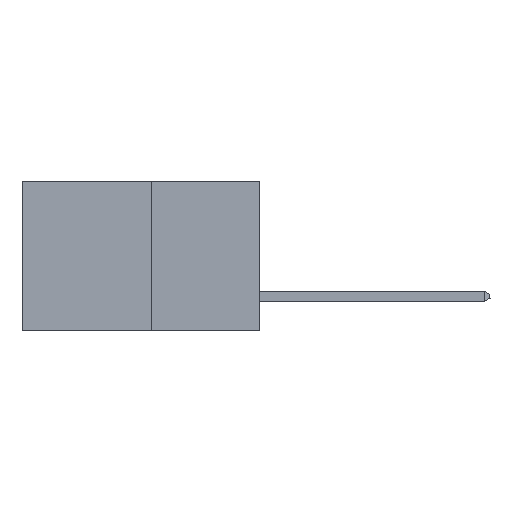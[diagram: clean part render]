
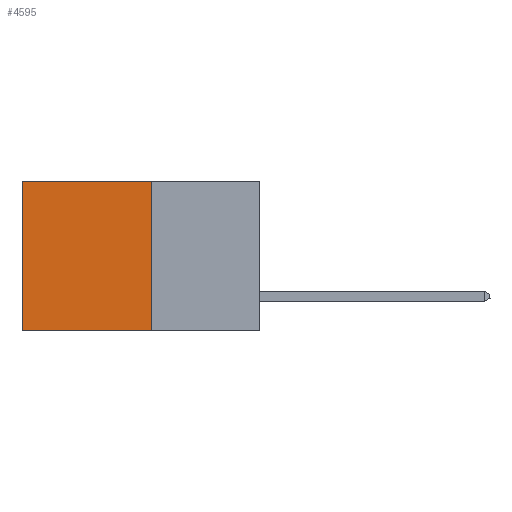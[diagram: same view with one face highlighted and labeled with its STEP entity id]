
A CAD part, left-side view. The second image highlights one B-rep face of the part: STEP entity #4595.
In plain terms, the highlighted planar face has unit normal (-1, 0, 0).
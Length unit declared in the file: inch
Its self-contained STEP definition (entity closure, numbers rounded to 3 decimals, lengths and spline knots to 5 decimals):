
#292 = VERTEX_POINT ( 'NONE', #19836 ) ;
#412 = VECTOR ( 'NONE', #15013, 39.37008 ) ;
#705 = VERTEX_POINT ( 'NONE', #16910 ) ;
#838 = EDGE_CURVE ( 'NONE', #19874, #292, #8129, .T. ) ;
#3374 = VECTOR ( 'NONE', #9735, 39.37008 ) ;
#4595 = ADVANCED_FACE ( 'NONE', ( #14822 ), #22034, .F. ) ;
#4630 = DIRECTION ( 'NONE',  ( 0., 0., -1. ) ) ;
#5185 = VECTOR ( 'NONE', #4630, 39.37008 ) ;
#5387 = CARTESIAN_POINT ( 'NONE',  ( 0.277, 0.27, -0.37 ) ) ;
#5677 = LINE ( 'NONE', #21864, #412 ) ;
#5822 = ORIENTED_EDGE ( 'NONE', *, *, #16742, .T. ) ;
#7137 = ORIENTED_EDGE ( 'NONE', *, *, #838, .F. ) ;
#7269 = VERTEX_POINT ( 'NONE', #12949 ) ;
#8129 = LINE ( 'NONE', #21641, #11764 ) ;
#8142 = LINE ( 'NONE', #21862, #3374 ) ;
#8742 = EDGE_CURVE ( 'NONE', #705, #7269, #8142, .T. ) ;
#9735 = DIRECTION ( 'NONE',  ( 0., 1., 0. ) ) ;
#10156 = ORIENTED_EDGE ( 'NONE', *, *, #8742, .T. ) ;
#10271 = EDGE_LOOP ( 'NONE', ( #5822, #7137, #12838, #10156 ) ) ;
#11761 = CARTESIAN_POINT ( 'NONE',  ( 0.277, 0.59, -0.37 ) ) ;
#11764 = VECTOR ( 'NONE', #19423, 39.37008 ) ;
#12110 = EDGE_CURVE ( 'NONE', #705, #19874, #5677, .T. ) ;
#12838 = ORIENTED_EDGE ( 'NONE', *, *, #12110, .F. ) ;
#12949 = CARTESIAN_POINT ( 'NONE',  ( 0.277, 0.59, 0. ) ) ;
#14618 = LINE ( 'NONE', #11761, #5185 ) ;
#14822 = FACE_OUTER_BOUND ( 'NONE', #10271, .T. ) ;
#15013 = DIRECTION ( 'NONE',  ( 0., 0., -1. ) ) ;
#16742 = EDGE_CURVE ( 'NONE', #7269, #292, #14618, .T. ) ;
#16910 = CARTESIAN_POINT ( 'NONE',  ( 0.277, 0.27, 0. ) ) ;
#16992 = AXIS2_PLACEMENT_3D ( 'NONE', #17439, #21465, #22270 ) ;
#17439 = CARTESIAN_POINT ( 'NONE',  ( 0.277, 0.27, -0.37 ) ) ;
#19423 = DIRECTION ( 'NONE',  ( 0., 1., 0. ) ) ;
#19836 = CARTESIAN_POINT ( 'NONE',  ( 0.277, 0.59, -0.37 ) ) ;
#19874 = VERTEX_POINT ( 'NONE', #5387 ) ;
#21465 = DIRECTION ( 'NONE',  ( 1., 0., 0. ) ) ;
#21641 = CARTESIAN_POINT ( 'NONE',  ( 0.277, 0.27, -0.37 ) ) ;
#21862 = CARTESIAN_POINT ( 'NONE',  ( 0.277, 0.27, 0. ) ) ;
#21864 = CARTESIAN_POINT ( 'NONE',  ( 0.277, 0.27, -0.37 ) ) ;
#22034 = PLANE ( 'NONE',  #16992 ) ;
#22270 = DIRECTION ( 'NONE',  ( 0., 0., -1. ) ) ;
